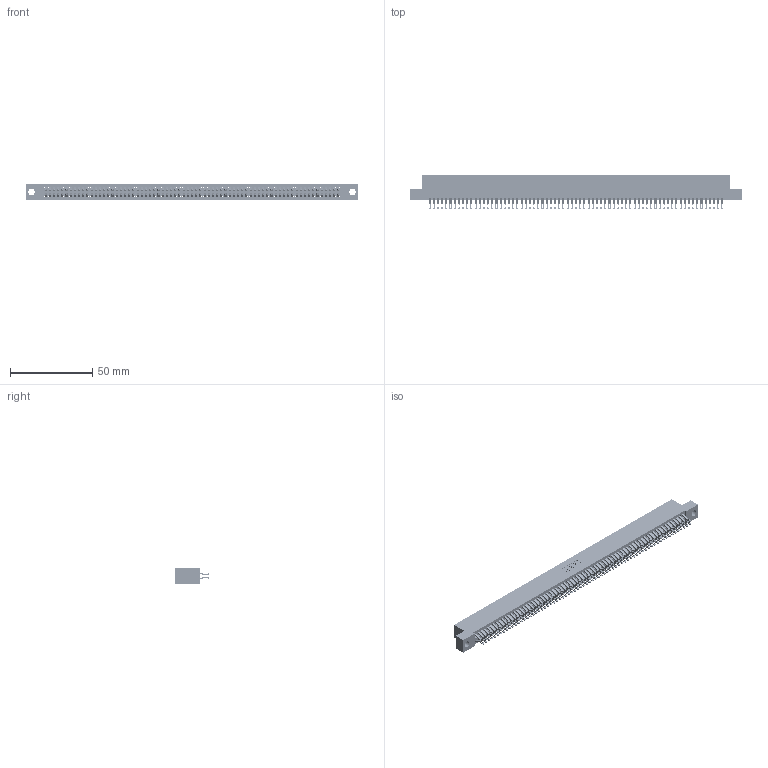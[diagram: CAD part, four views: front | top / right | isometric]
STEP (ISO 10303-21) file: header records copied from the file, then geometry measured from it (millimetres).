
FILE_DESCRIPTION (( 'STEP AP203' ), '1' );
FILE_NAME ('395-142-555-204.STEP', '2018-12-06T03:42:58', ( '' ), ( '' ), 'SwSTEP 2.0', 'SolidWorks 2016', '' );
FILE_SCHEMA (( 'CONFIG_CONTROL_DESIGN' ));
Length unit declared in the file: inch
Products named in the file (3): 395-142-555-204; 345-292-001_555 Tail; 345 Part_Flush Mounting Lugs - 0.156 Dia-TH
Assembly tree (143 placements, depth 2):
  395-142-555-204
    345 Part_Flush Mounting Lugs - 0.156 Dia-TH
    345-292-001_555 Tail  x142
Bounding box: 201.55 x 21.13 x 9.4 mm (x, y, z)
Volume: 20171.9 mm3; surface area: 31626.8 mm2
Topology: 143 solids, 143 shells, 8078 faces, 25475 edges, 16982 vertices
Faces by surface type: plane 4482, cylinder 3596
Entity records: 52133 total; most frequent: CARTESIAN_POINT 8746, ORIENTED_EDGE 8650, DIRECTION 7645, EDGE_CURVE 4325, LINE 3889, VECTOR 3889, VERTEX_POINT 2882, AXIS2_PLACEMENT_3D 1878
